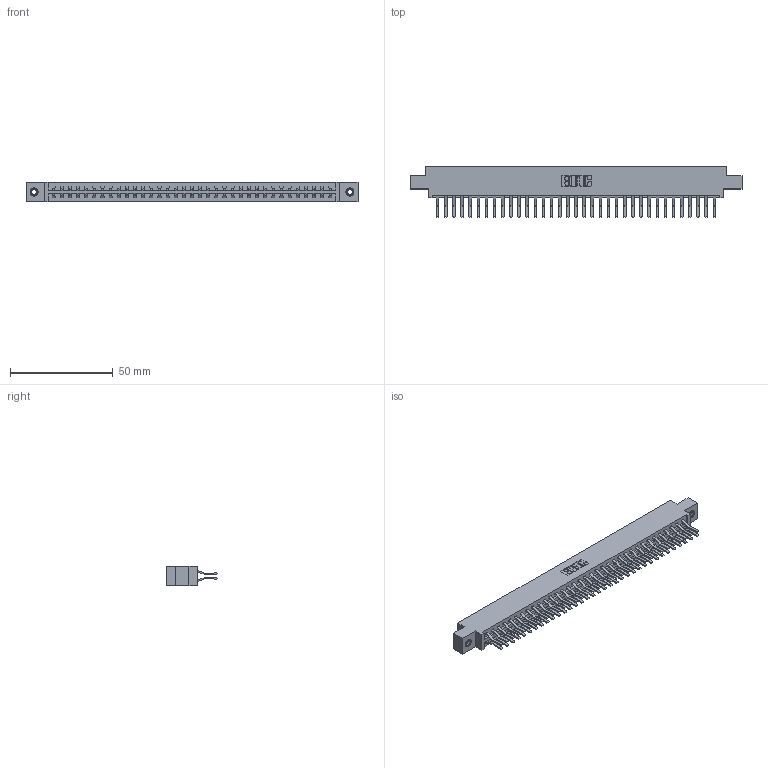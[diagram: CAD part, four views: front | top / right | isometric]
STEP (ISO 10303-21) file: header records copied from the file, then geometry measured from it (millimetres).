
FILE_DESCRIPTION (( 'STEP AP203' ), '1' );
FILE_NAME ('337-070-560-807.STEP', '2019-10-15T11:20:22', ( '' ), ( '' ), 'SwSTEP 2.0', 'SolidWorks 2016', '' );
FILE_SCHEMA (( 'CONFIG_CONTROL_DESIGN' ));
Length unit declared in the file: inch
Products named in the file (4): 345-292-001_560 Tail; 337 Part_0.170 Offset - 0.156 Dia-TI; 337-070-560-807; 345-250-001_345-250-005-103
Assembly tree (73 placements, depth 2):
  337-070-560-807
    337 Part_0.170 Offset - 0.156 Dia-TI
    345-292-001_560 Tail  x70
    345-250-001_345-250-005-103  x2
Bounding box: 161.7 x 24.78 x 9.4 mm (x, y, z)
Volume: 17275.5 mm3; surface area: 20933.7 mm2
Topology: 73 solids, 73 shells, 4098 faces, 12149 edges, 7998 vertices
Faces by surface type: plane 2766, cylinder 1316, cone 12, torus 4
Entity records: 29448 total; most frequent: CARTESIAN_POINT 4949, ORIENTED_EDGE 4878, DIRECTION 4257, EDGE_CURVE 2439, VECTOR 2287, LINE 2287, VERTEX_POINT 1620, AXIS2_PLACEMENT_3D 985
